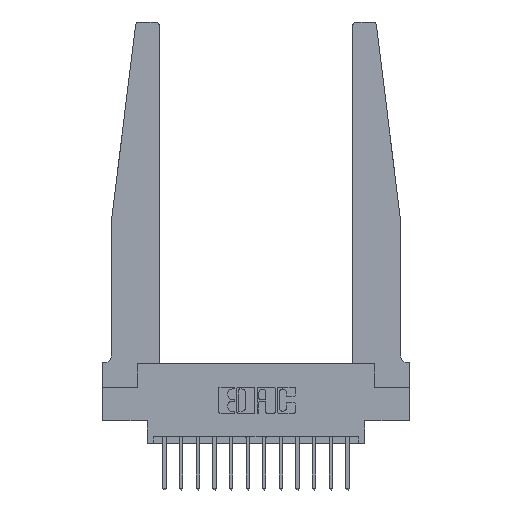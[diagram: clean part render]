
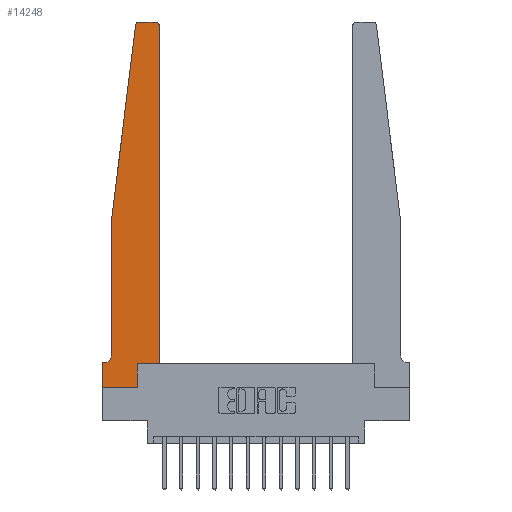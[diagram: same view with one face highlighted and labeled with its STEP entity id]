
A CAD part, top view. The second image highlights one B-rep face of the part: STEP entity #14248.
In plain terms, the highlighted planar face has unit normal (0, 0, 1).
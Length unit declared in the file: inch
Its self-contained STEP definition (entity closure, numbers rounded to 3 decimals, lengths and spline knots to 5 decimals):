
#472 = DIRECTION ( 'NONE',  ( 1., 0., 0. ) ) ;
#537 = CIRCLE ( 'NONE', #11665, 0.03 ) ;
#1037 = CARTESIAN_POINT ( 'NONE',  ( 0.065, 0.1875, 0.37 ) ) ;
#1294 = VERTEX_POINT ( 'NONE', #15099 ) ;
#1407 = CARTESIAN_POINT ( 'NONE',  ( 0.24675, 2.72367, 0.37 ) ) ;
#1499 = DIRECTION ( 'NONE',  ( 1., 0., 0. ) ) ;
#1575 = DIRECTION ( 'NONE',  ( 0., -1., 0. ) ) ;
#2021 = PLANE ( 'NONE',  #11659 ) ;
#2402 = LINE ( 'NONE', #5166, #12996 ) ;
#2440 = VERTEX_POINT ( 'NONE', #13559 ) ;
#2543 = VECTOR ( 'NONE', #1499, 39.37008 ) ;
#2726 = LINE ( 'NONE', #2901, #9115 ) ;
#2901 = CARTESIAN_POINT ( 'NONE',  ( 0.2605, 0.18, 0.37 ) ) ;
#2917 = ORIENTED_EDGE ( 'NONE', *, *, #11973, .T. ) ;
#2993 = LINE ( 'NONE', #8303, #13027 ) ;
#3115 = CARTESIAN_POINT ( 'NONE',  ( 0.015, 0.1875, 0.37 ) ) ;
#3195 = CARTESIAN_POINT ( 'NONE',  ( 0., 0., 0.37 ) ) ;
#3399 = VERTEX_POINT ( 'NONE', #4283 ) ;
#3434 = CARTESIAN_POINT ( 'NONE',  ( 0.395, 2.72, 0.37 ) ) ;
#4128 = VECTOR ( 'NONE', #4975, 39.37008 ) ;
#4152 = ORIENTED_EDGE ( 'NONE', *, *, #16932, .T. ) ;
#4195 = ORIENTED_EDGE ( 'NONE', *, *, #17032, .T. ) ;
#4213 = DIRECTION ( 'NONE',  ( -0.122, -0.992, 0. ) ) ;
#4283 = CARTESIAN_POINT ( 'NONE',  ( 0.425, 2.72, 0.37 ) ) ;
#4634 = EDGE_CURVE ( 'NONE', #10109, #8124, #2993, .T. ) ;
#4776 = FACE_OUTER_BOUND ( 'NONE', #14931, .T. ) ;
#4882 = LINE ( 'NONE', #10362, #4128 ) ;
#4975 = DIRECTION ( 'NONE',  ( -1., 0., 0. ) ) ;
#5010 = LINE ( 'NONE', #11541, #5035 ) ;
#5035 = VECTOR ( 'NONE', #5274, 39.37008 ) ;
#5084 = LINE ( 'NONE', #10388, #7761 ) ;
#5166 = CARTESIAN_POINT ( 'NONE',  ( 0.425, 0.18, 0.37 ) ) ;
#5274 = DIRECTION ( 'NONE',  ( 1., 0., 0. ) ) ;
#5324 = ORIENTED_EDGE ( 'NONE', *, *, #15200, .T. ) ;
#5343 = EDGE_CURVE ( 'NONE', #3399, #16951, #537, .T. ) ;
#5373 = ORIENTED_EDGE ( 'NONE', *, *, #5343, .T. ) ;
#5399 = EDGE_CURVE ( 'NONE', #8124, #1294, #5084, .T. ) ;
#5604 = ORIENTED_EDGE ( 'NONE', *, *, #10206, .T. ) ;
#5760 = EDGE_CURVE ( 'NONE', #13324, #10109, #11675, .T. ) ;
#6270 = DIRECTION ( 'NONE',  ( 1., 0., 0. ) ) ;
#6318 = DIRECTION ( 'NONE',  ( 0., -1., 0. ) ) ;
#6338 = LINE ( 'NONE', #1037, #12294 ) ;
#6640 = VERTEX_POINT ( 'NONE', #13362 ) ;
#6659 = CARTESIAN_POINT ( 'NONE',  ( 0., 0., 0.37 ) ) ;
#7066 = ORIENTED_EDGE ( 'NONE', *, *, #4634, .T. ) ;
#7431 = VERTEX_POINT ( 'NONE', #3115 ) ;
#7581 = CARTESIAN_POINT ( 'NONE',  ( 0., 0.1875, 0.37 ) ) ;
#7727 = EDGE_CURVE ( 'NONE', #6640, #8010, #5010, .T. ) ;
#7761 = VECTOR ( 'NONE', #6318, 39.37008 ) ;
#7785 = CARTESIAN_POINT ( 'NONE',  ( 0.065, 1.25, 0.37 ) ) ;
#8010 = VERTEX_POINT ( 'NONE', #9686 ) ;
#8011 = CARTESIAN_POINT ( 'NONE',  ( 0., 0., 0.37 ) ) ;
#8124 = VERTEX_POINT ( 'NONE', #7785 ) ;
#8133 = DIRECTION ( 'NONE',  ( -1., 0., 0. ) ) ;
#8303 = CARTESIAN_POINT ( 'NONE',  ( 0.065, 1.25, 0.37 ) ) ;
#8313 = DIRECTION ( 'NONE',  ( 0., 0., 1. ) ) ;
#8908 = EDGE_CURVE ( 'NONE', #7431, #15101, #6338, .T. ) ;
#9115 = VECTOR ( 'NONE', #17082, 39.37008 ) ;
#9606 = ORIENTED_EDGE ( 'NONE', *, *, #11894, .T. ) ;
#9678 = CARTESIAN_POINT ( 'NONE',  ( 0.27653, 2.72, 0.37 ) ) ;
#9686 = CARTESIAN_POINT ( 'NONE',  ( 0.425, 0.18, 0.37 ) ) ;
#9755 = VERTEX_POINT ( 'NONE', #6659 ) ;
#10109 = VERTEX_POINT ( 'NONE', #1407 ) ;
#10206 = EDGE_CURVE ( 'NONE', #9755, #2440, #11024, .T. ) ;
#10362 = CARTESIAN_POINT ( 'NONE',  ( 0.25, 2.75, 0.37 ) ) ;
#10388 = CARTESIAN_POINT ( 'NONE',  ( 0.065, 1.25, 0.37 ) ) ;
#11024 = LINE ( 'NONE', #8011, #2543 ) ;
#11191 = CARTESIAN_POINT ( 'NONE',  ( 0.27653, 2.75, 0.37 ) ) ;
#11541 = CARTESIAN_POINT ( 'NONE',  ( 0.425, 0.18, 0.37 ) ) ;
#11659 = AXIS2_PLACEMENT_3D ( 'NONE', #7581, #12619, #6270 ) ;
#11665 = AXIS2_PLACEMENT_3D ( 'NONE', #3434, #15533, #17021 ) ;
#11675 = CIRCLE ( 'NONE', #12496, 0.03 ) ;
#11894 = EDGE_CURVE ( 'NONE', #15101, #9755, #13482, .T. ) ;
#11973 = EDGE_CURVE ( 'NONE', #8010, #3399, #2402, .T. ) ;
#12264 = ORIENTED_EDGE ( 'NONE', *, *, #5760, .T. ) ;
#12294 = VECTOR ( 'NONE', #14183, 39.37008 ) ;
#12496 = AXIS2_PLACEMENT_3D ( 'NONE', #9678, #8313, #472 ) ;
#12619 = DIRECTION ( 'NONE',  ( 0., 0., 1. ) ) ;
#12746 = ORIENTED_EDGE ( 'NONE', *, *, #5399, .T. ) ;
#12996 = VECTOR ( 'NONE', #14155, 39.37008 ) ;
#13027 = VECTOR ( 'NONE', #4213, 39.37008 ) ;
#13079 = DIRECTION ( 'NONE',  ( 0., 0., -1. ) ) ;
#13324 = VERTEX_POINT ( 'NONE', #11191 ) ;
#13362 = CARTESIAN_POINT ( 'NONE',  ( 0.2605, 0.18, 0.37 ) ) ;
#13482 = LINE ( 'NONE', #3195, #16058 ) ;
#13513 = AXIS2_PLACEMENT_3D ( 'NONE', #14403, #13079, #8133 ) ;
#13559 = CARTESIAN_POINT ( 'NONE',  ( 0.2605, 0., 0.37 ) ) ;
#14155 = DIRECTION ( 'NONE',  ( 0., 1., 0. ) ) ;
#14176 = ORIENTED_EDGE ( 'NONE', *, *, #7727, .T. ) ;
#14183 = DIRECTION ( 'NONE',  ( -1., 0., 0. ) ) ;
#14248 = ADVANCED_FACE ( 'NONE', ( #4776 ), #2021, .T. ) ;
#14403 = CARTESIAN_POINT ( 'NONE',  ( 0.015, 0.2375, 0.37 ) ) ;
#14931 = EDGE_LOOP ( 'NONE', ( #4152, #12264, #7066, #12746, #5324, #16485, #9606, #5604, #4195, #14176, #2917, #5373 ) ) ;
#15099 = CARTESIAN_POINT ( 'NONE',  ( 0.065, 0.2375, 0.37 ) ) ;
#15101 = VERTEX_POINT ( 'NONE', #15414 ) ;
#15200 = EDGE_CURVE ( 'NONE', #1294, #7431, #17125, .T. ) ;
#15414 = CARTESIAN_POINT ( 'NONE',  ( 0., 0.1875, 0.37 ) ) ;
#15533 = DIRECTION ( 'NONE',  ( 0., 0., 1. ) ) ;
#16058 = VECTOR ( 'NONE', #1575, 39.37008 ) ;
#16485 = ORIENTED_EDGE ( 'NONE', *, *, #8908, .T. ) ;
#16932 = EDGE_CURVE ( 'NONE', #16951, #13324, #4882, .T. ) ;
#16951 = VERTEX_POINT ( 'NONE', #16995 ) ;
#16995 = CARTESIAN_POINT ( 'NONE',  ( 0.395, 2.75, 0.37 ) ) ;
#17021 = DIRECTION ( 'NONE',  ( 1., 0., 0. ) ) ;
#17032 = EDGE_CURVE ( 'NONE', #2440, #6640, #2726, .T. ) ;
#17082 = DIRECTION ( 'NONE',  ( 0., 1., 0. ) ) ;
#17125 = CIRCLE ( 'NONE', #13513, 0.05 ) ;
